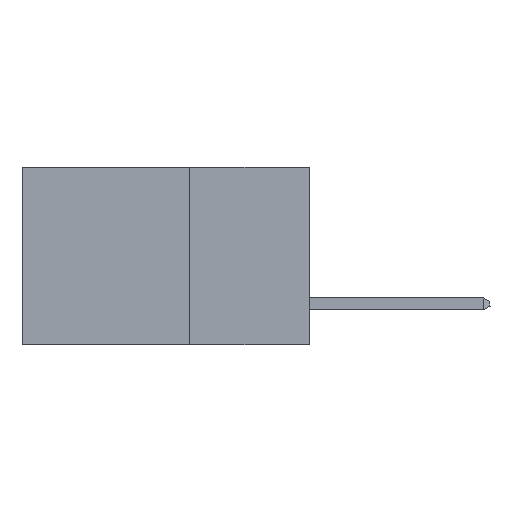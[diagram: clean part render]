
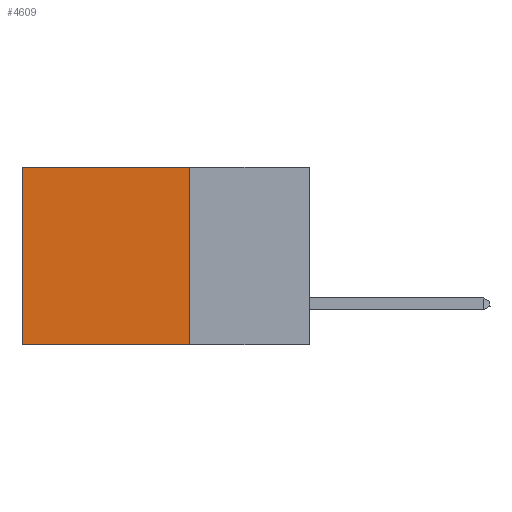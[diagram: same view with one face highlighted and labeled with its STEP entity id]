
A CAD part, left-side view. The second image highlights one B-rep face of the part: STEP entity #4609.
In plain terms, the highlighted planar face has unit normal (-1, 0, 0).
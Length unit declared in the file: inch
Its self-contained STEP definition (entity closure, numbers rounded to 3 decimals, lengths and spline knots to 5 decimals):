
#34 = PLANE ( 'NONE',  #7216 ) ;
#345 = VERTEX_POINT ( 'NONE', #4815 ) ;
#450 = CARTESIAN_POINT ( 'NONE',  ( 0.2875, 0.6, 0. ) ) ;
#495 = VERTEX_POINT ( 'NONE', #450 ) ;
#1116 = VERTEX_POINT ( 'NONE', #2561 ) ;
#1481 = DIRECTION ( 'NONE',  ( 0., 1., 0. ) ) ;
#1539 = EDGE_LOOP ( 'NONE', ( #9273, #5562, #8325, #5927 ) ) ;
#2561 = CARTESIAN_POINT ( 'NONE',  ( 0.2875, 0.6, -0.37 ) ) ;
#3140 = DIRECTION ( 'NONE',  ( 0., 0., -1. ) ) ;
#3591 = VECTOR ( 'NONE', #1481, 39.37008 ) ;
#3863 = EDGE_CURVE ( 'NONE', #345, #9699, #11263, .T. ) ;
#3904 = VECTOR ( 'NONE', #9154, 39.37008 ) ;
#4609 = ADVANCED_FACE ( 'NONE', ( #6937 ), #34, .F. ) ;
#4815 = CARTESIAN_POINT ( 'NONE',  ( 0.2875, 0.25, 0. ) ) ;
#5078 = CARTESIAN_POINT ( 'NONE',  ( 0.2875, 0.25, -0.37 ) ) ;
#5144 = DIRECTION ( 'NONE',  ( 1., 0., 0. ) ) ;
#5170 = CARTESIAN_POINT ( 'NONE',  ( 0.2875, 0.25, 0. ) ) ;
#5562 = ORIENTED_EDGE ( 'NONE', *, *, #7440, .F. ) ;
#5927 = ORIENTED_EDGE ( 'NONE', *, *, #9557, .T. ) ;
#6532 = LINE ( 'NONE', #9466, #10990 ) ;
#6541 = LINE ( 'NONE', #5078, #3904 ) ;
#6937 = FACE_OUTER_BOUND ( 'NONE', #1539, .T. ) ;
#7216 = AXIS2_PLACEMENT_3D ( 'NONE', #11646, #5144, #8348 ) ;
#7440 = EDGE_CURVE ( 'NONE', #9699, #1116, #6541, .T. ) ;
#8214 = LINE ( 'NONE', #13050, #3591 ) ;
#8325 = ORIENTED_EDGE ( 'NONE', *, *, #3863, .F. ) ;
#8348 = DIRECTION ( 'NONE',  ( 0., 0., -1. ) ) ;
#9154 = DIRECTION ( 'NONE',  ( 0., 1., 0. ) ) ;
#9273 = ORIENTED_EDGE ( 'NONE', *, *, #10554, .T. ) ;
#9466 = CARTESIAN_POINT ( 'NONE',  ( 0.2875, 0.6, 0. ) ) ;
#9557 = EDGE_CURVE ( 'NONE', #345, #495, #8214, .T. ) ;
#9699 = VERTEX_POINT ( 'NONE', #10311 ) ;
#10311 = CARTESIAN_POINT ( 'NONE',  ( 0.2875, 0.25, -0.37 ) ) ;
#10554 = EDGE_CURVE ( 'NONE', #495, #1116, #6532, .T. ) ;
#10990 = VECTOR ( 'NONE', #3140, 39.37008 ) ;
#11263 = LINE ( 'NONE', #5170, #13566 ) ;
#11646 = CARTESIAN_POINT ( 'NONE',  ( 0.2875, 0.25, 0. ) ) ;
#13050 = CARTESIAN_POINT ( 'NONE',  ( 0.2875, 0.25, 0. ) ) ;
#13566 = VECTOR ( 'NONE', #13575, 39.37008 ) ;
#13575 = DIRECTION ( 'NONE',  ( 0., 0., -1. ) ) ;
